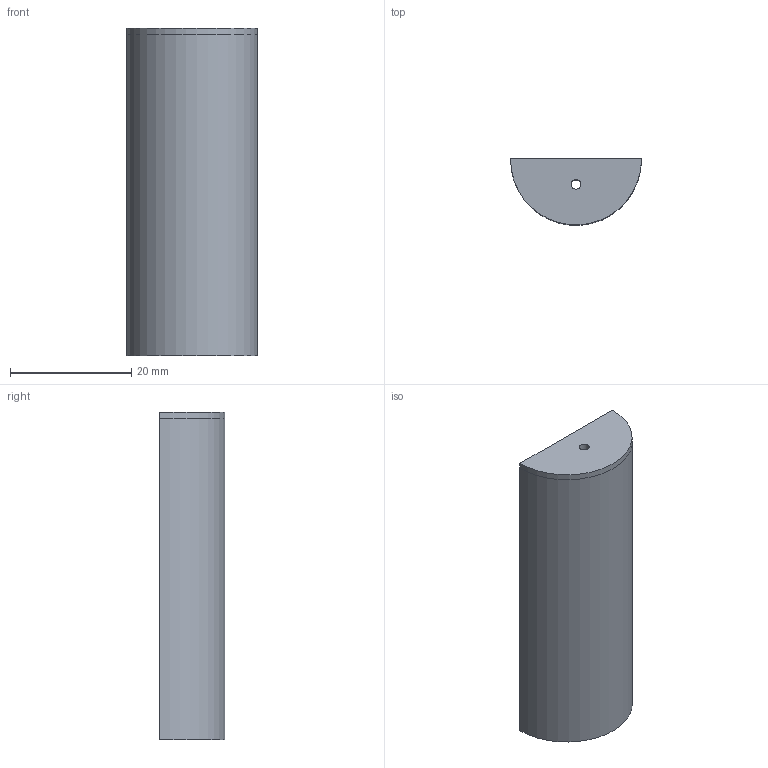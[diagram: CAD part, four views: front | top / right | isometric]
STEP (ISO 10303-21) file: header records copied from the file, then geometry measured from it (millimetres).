
FILE_DESCRIPTION(('FreeCAD Model'),'2;1');
FILE_NAME('WTF-9 firing pin jig.step', '2020-05-12T16:19:37',('Author'),(''), 'Open CASCADE STEP processor 6.8','FreeCAD','Unknown');
FILE_SCHEMA(('AUTOMOTIVE_DESIGN_CC2 { 1 2 10303 214 -1 1 5 4 }'));
Length unit declared in the file: millimetre
Products named in the file (1): Pocket002
Bounding box: 21.6 x 10.89 x 54 mm (x, y, z)
Volume: 2253.1 mm3; surface area: 4272.8 mm2
Topology: 1 solids, 1 shells, 13 faces, 29 edges, 19 vertices
Faces by surface type: cylinder 8, plane 5
Full cylindrical faces by diameter (mm): 1.6 x2
Entity records: 793 total; most frequent: CARTESIAN_POINT 210, DIRECTION 99, ORIENTED_EDGE 58, PCURVE 58, DEFINITIONAL_REPRESENTATION 58, LINE 43, VECTOR 43, EDGE_CURVE 29
